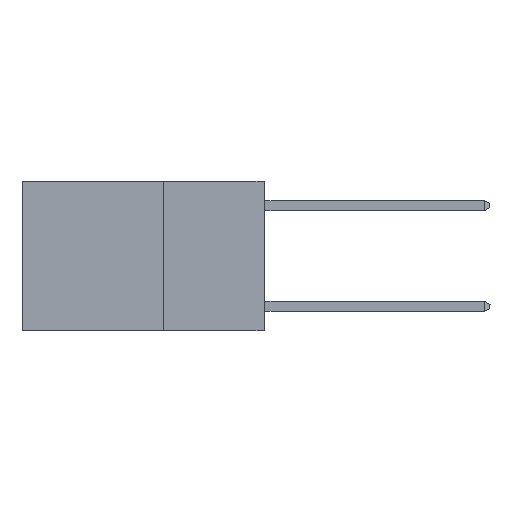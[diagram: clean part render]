
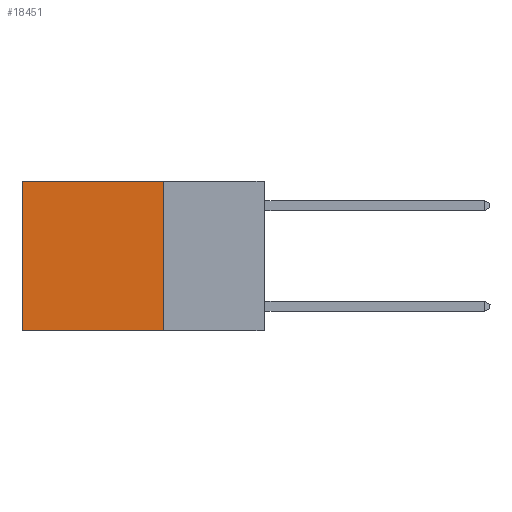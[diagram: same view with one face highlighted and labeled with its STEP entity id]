
A CAD part, left-side view. The second image highlights one B-rep face of the part: STEP entity #18451.
In plain terms, the highlighted planar face has unit normal (-1, 0, 0).
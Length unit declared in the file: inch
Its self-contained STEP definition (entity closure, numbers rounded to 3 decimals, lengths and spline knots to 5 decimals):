
#580 = LINE ( 'NONE', #4730, #22669 ) ;
#893 = VERTEX_POINT ( 'NONE', #3517 ) ;
#1173 = DIRECTION ( 'NONE',  ( 0., 0., -1. ) ) ;
#3517 = CARTESIAN_POINT ( 'NONE',  ( 0.2625, 0.25, -0.37 ) ) ;
#4593 = FACE_OUTER_BOUND ( 'NONE', #17229, .T. ) ;
#4730 = CARTESIAN_POINT ( 'NONE',  ( 0.2625, 0.6, 0. ) ) ;
#5722 = LINE ( 'NONE', #16242, #10077 ) ;
#6247 = PLANE ( 'NONE',  #26907 ) ;
#6498 = CARTESIAN_POINT ( 'NONE',  ( 0.2625, 0.6, 0. ) ) ;
#7421 = ORIENTED_EDGE ( 'NONE', *, *, #27334, .F. ) ;
#7425 = CARTESIAN_POINT ( 'NONE',  ( 0.2625, 0.25, 0. ) ) ;
#7724 = CARTESIAN_POINT ( 'NONE',  ( 0.2625, 0.25, 0. ) ) ;
#7948 = VECTOR ( 'NONE', #15440, 39.37008 ) ;
#8406 = CARTESIAN_POINT ( 'NONE',  ( 0.2625, 0.25, 0. ) ) ;
#8414 = VECTOR ( 'NONE', #20215, 39.37008 ) ;
#10077 = VECTOR ( 'NONE', #1173, 39.37008 ) ;
#10526 = DIRECTION ( 'NONE',  ( 1., 0., 0. ) ) ;
#13587 = LINE ( 'NONE', #17305, #7948 ) ;
#13621 = VERTEX_POINT ( 'NONE', #19369 ) ;
#14080 = LINE ( 'NONE', #7425, #8414 ) ;
#15440 = DIRECTION ( 'NONE',  ( 0., 1., 0. ) ) ;
#15488 = EDGE_CURVE ( 'NONE', #25055, #19184, #14080, .T. ) ;
#16242 = CARTESIAN_POINT ( 'NONE',  ( 0.2625, 0.25, 0. ) ) ;
#17229 = EDGE_LOOP ( 'NONE', ( #25961, #7421, #19076, #25114 ) ) ;
#17305 = CARTESIAN_POINT ( 'NONE',  ( 0.2625, 0.25, -0.37 ) ) ;
#18451 = ADVANCED_FACE ( 'NONE', ( #4593 ), #6247, .F. ) ;
#18608 = EDGE_CURVE ( 'NONE', #19184, #13621, #580, .T. ) ;
#19076 = ORIENTED_EDGE ( 'NONE', *, *, #22406, .F. ) ;
#19184 = VERTEX_POINT ( 'NONE', #6498 ) ;
#19369 = CARTESIAN_POINT ( 'NONE',  ( 0.2625, 0.6, -0.37 ) ) ;
#19711 = DIRECTION ( 'NONE',  ( 0., 0., -1. ) ) ;
#20215 = DIRECTION ( 'NONE',  ( 0., 1., 0. ) ) ;
#22406 = EDGE_CURVE ( 'NONE', #25055, #893, #5722, .T. ) ;
#22669 = VECTOR ( 'NONE', #19711, 39.37008 ) ;
#25055 = VERTEX_POINT ( 'NONE', #7724 ) ;
#25114 = ORIENTED_EDGE ( 'NONE', *, *, #15488, .T. ) ;
#25458 = DIRECTION ( 'NONE',  ( 0., 0., -1. ) ) ;
#25961 = ORIENTED_EDGE ( 'NONE', *, *, #18608, .T. ) ;
#26907 = AXIS2_PLACEMENT_3D ( 'NONE', #8406, #10526, #25458 ) ;
#27334 = EDGE_CURVE ( 'NONE', #893, #13621, #13587, .T. ) ;
